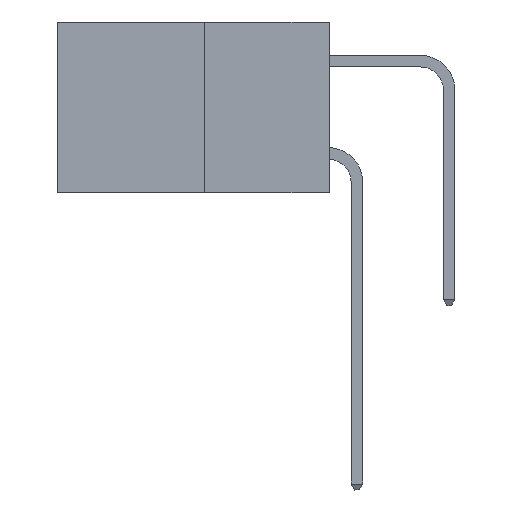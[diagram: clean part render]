
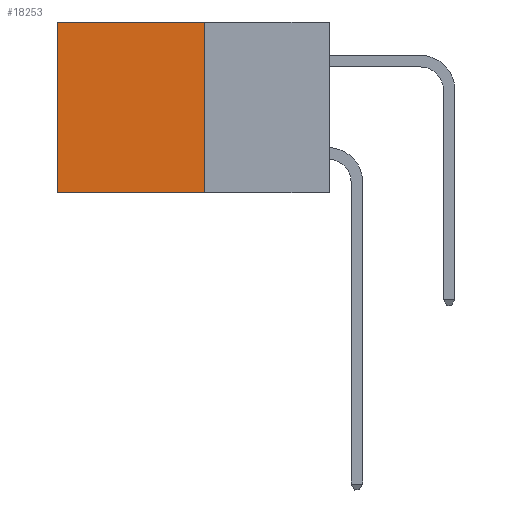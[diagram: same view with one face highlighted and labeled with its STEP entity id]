
A CAD part, left-side view. The second image highlights one B-rep face of the part: STEP entity #18253.
In plain terms, the highlighted planar face has unit normal (-1, 0, 0).
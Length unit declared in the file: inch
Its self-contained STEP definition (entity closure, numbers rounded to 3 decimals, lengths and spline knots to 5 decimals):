
#435 = LINE ( 'NONE', #6806, #17152 ) ;
#486 = DIRECTION ( 'NONE',  ( 0., 0., -1. ) ) ;
#2213 = CARTESIAN_POINT ( 'NONE',  ( 0.277, 0.27, -0.37 ) ) ;
#2228 = EDGE_CURVE ( 'NONE', #7736, #14978, #11157, .T. ) ;
#2326 = ORIENTED_EDGE ( 'NONE', *, *, #15787, .F. ) ;
#2675 = LINE ( 'NONE', #14842, #10433 ) ;
#3399 = DIRECTION ( 'NONE',  ( 0., 1., 0. ) ) ;
#3845 = DIRECTION ( 'NONE',  ( 0., 0., -1. ) ) ;
#4558 = EDGE_CURVE ( 'NONE', #5898, #7840, #2675, .T. ) ;
#5408 = LINE ( 'NONE', #15745, #16850 ) ;
#5898 = VERTEX_POINT ( 'NONE', #10726 ) ;
#6806 = CARTESIAN_POINT ( 'NONE',  ( 0.277, 0.27, 0. ) ) ;
#6824 = DIRECTION ( 'NONE',  ( 0., 1., 0. ) ) ;
#7727 = FACE_OUTER_BOUND ( 'NONE', #11086, .T. ) ;
#7736 = VERTEX_POINT ( 'NONE', #19762 ) ;
#7840 = VERTEX_POINT ( 'NONE', #12357 ) ;
#8109 = ORIENTED_EDGE ( 'NONE', *, *, #4558, .T. ) ;
#8374 = ORIENTED_EDGE ( 'NONE', *, *, #2228, .F. ) ;
#8820 = AXIS2_PLACEMENT_3D ( 'NONE', #11556, #13131, #3845 ) ;
#9600 = ORIENTED_EDGE ( 'NONE', *, *, #12360, .T. ) ;
#10027 = PLANE ( 'NONE',  #8820 ) ;
#10133 = CARTESIAN_POINT ( 'NONE',  ( 0.277, 0.27, -0.37 ) ) ;
#10433 = VECTOR ( 'NONE', #486, 39.37008 ) ;
#10726 = CARTESIAN_POINT ( 'NONE',  ( 0.277, 0.59, 0. ) ) ;
#11086 = EDGE_LOOP ( 'NONE', ( #8109, #2326, #8374, #9600 ) ) ;
#11157 = LINE ( 'NONE', #10133, #18909 ) ;
#11556 = CARTESIAN_POINT ( 'NONE',  ( 0.277, 0.27, -0.37 ) ) ;
#12357 = CARTESIAN_POINT ( 'NONE',  ( 0.277, 0.59, -0.37 ) ) ;
#12360 = EDGE_CURVE ( 'NONE', #7736, #5898, #435, .T. ) ;
#13131 = DIRECTION ( 'NONE',  ( 1., 0., 0. ) ) ;
#14842 = CARTESIAN_POINT ( 'NONE',  ( 0.277, 0.59, -0.37 ) ) ;
#14978 = VERTEX_POINT ( 'NONE', #2213 ) ;
#15745 = CARTESIAN_POINT ( 'NONE',  ( 0.277, 0.27, -0.37 ) ) ;
#15787 = EDGE_CURVE ( 'NONE', #14978, #7840, #5408, .T. ) ;
#16045 = DIRECTION ( 'NONE',  ( 0., 0., -1. ) ) ;
#16850 = VECTOR ( 'NONE', #3399, 39.37008 ) ;
#17152 = VECTOR ( 'NONE', #6824, 39.37008 ) ;
#18253 = ADVANCED_FACE ( 'NONE', ( #7727 ), #10027, .F. ) ;
#18909 = VECTOR ( 'NONE', #16045, 39.37008 ) ;
#19762 = CARTESIAN_POINT ( 'NONE',  ( 0.277, 0.27, 0. ) ) ;
